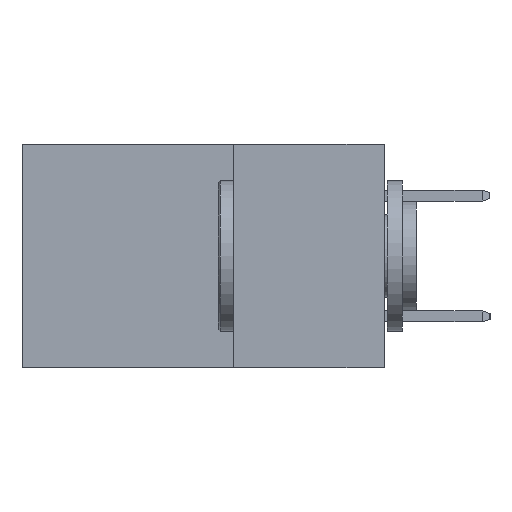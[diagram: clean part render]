
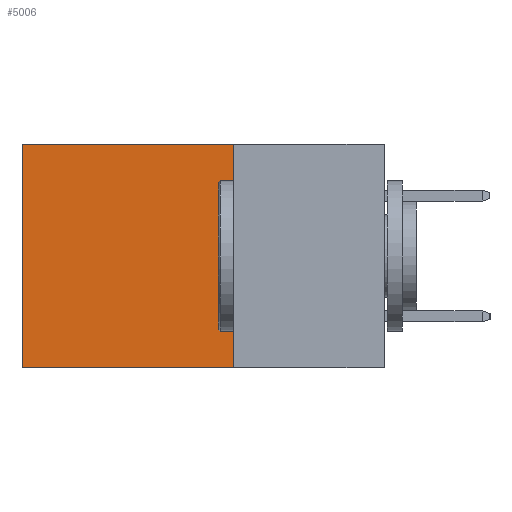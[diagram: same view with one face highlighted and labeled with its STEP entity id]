
A CAD part, left-side view. The second image highlights one B-rep face of the part: STEP entity #5006.
In plain terms, the highlighted planar face has unit normal (-1, 0, 0).
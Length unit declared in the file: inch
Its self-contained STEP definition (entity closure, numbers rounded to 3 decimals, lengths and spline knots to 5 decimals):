
#15 = DIRECTION ( 'NONE',  ( 0., 1., 0. ) ) ;
#39 = CARTESIAN_POINT ( 'NONE',  ( 0.2615, 0.25, -0.37 ) ) ;
#132 = CARTESIAN_POINT ( 'NONE',  ( 0.2615, 0.6, -0.37 ) ) ;
#554 = AXIS2_PLACEMENT_3D ( 'NONE', #7842, #7624, #7474 ) ;
#948 = EDGE_CURVE ( 'NONE', #9832, #2576, #1438, .T. ) ;
#1438 = LINE ( 'NONE', #8439, #6873 ) ;
#1490 = CARTESIAN_POINT ( 'NONE',  ( 0.2615, 0.6, -0.37 ) ) ;
#1623 = DIRECTION ( 'NONE',  ( 0., 0., -1. ) ) ;
#2576 = VERTEX_POINT ( 'NONE', #8245 ) ;
#2884 = VERTEX_POINT ( 'NONE', #132 ) ;
#3644 = ORIENTED_EDGE ( 'NONE', *, *, #8333, .T. ) ;
#3661 = DIRECTION ( 'NONE',  ( 0., 1., 0. ) ) ;
#3994 = CARTESIAN_POINT ( 'NONE',  ( 0.2615, 0.25, 0. ) ) ;
#4222 = EDGE_CURVE ( 'NONE', #2576, #2884, #5052, .T. ) ;
#4722 = VECTOR ( 'NONE', #15, 39.37008 ) ;
#5006 = ADVANCED_FACE ( 'NONE', ( #12480 ), #7931, .F. ) ;
#5024 = LINE ( 'NONE', #1490, #10415 ) ;
#5052 = LINE ( 'NONE', #39, #4722 ) ;
#5060 = CARTESIAN_POINT ( 'NONE',  ( 0.2615, 0.6, 0. ) ) ;
#5174 = EDGE_CURVE ( 'NONE', #12425, #2884, #5024, .T. ) ;
#5870 = ORIENTED_EDGE ( 'NONE', *, *, #4222, .F. ) ;
#6322 = CARTESIAN_POINT ( 'NONE',  ( 0.2615, 0.25, 0. ) ) ;
#6873 = VECTOR ( 'NONE', #7033, 39.37008 ) ;
#7033 = DIRECTION ( 'NONE',  ( 0., 0., -1. ) ) ;
#7474 = DIRECTION ( 'NONE',  ( 0., 0., -1. ) ) ;
#7513 = ORIENTED_EDGE ( 'NONE', *, *, #948, .F. ) ;
#7514 = EDGE_LOOP ( 'NONE', ( #11920, #5870, #7513, #3644 ) ) ;
#7624 = DIRECTION ( 'NONE',  ( 1., 0., 0. ) ) ;
#7842 = CARTESIAN_POINT ( 'NONE',  ( 0.2615, 0.25, -0.37 ) ) ;
#7931 = PLANE ( 'NONE',  #554 ) ;
#8245 = CARTESIAN_POINT ( 'NONE',  ( 0.2615, 0.25, -0.37 ) ) ;
#8333 = EDGE_CURVE ( 'NONE', #9832, #12425, #11278, .T. ) ;
#8403 = VECTOR ( 'NONE', #3661, 39.37008 ) ;
#8439 = CARTESIAN_POINT ( 'NONE',  ( 0.2615, 0.25, -0.37 ) ) ;
#9832 = VERTEX_POINT ( 'NONE', #6322 ) ;
#10415 = VECTOR ( 'NONE', #1623, 39.37008 ) ;
#11278 = LINE ( 'NONE', #3994, #8403 ) ;
#11920 = ORIENTED_EDGE ( 'NONE', *, *, #5174, .T. ) ;
#12425 = VERTEX_POINT ( 'NONE', #5060 ) ;
#12480 = FACE_OUTER_BOUND ( 'NONE', #7514, .T. ) ;
